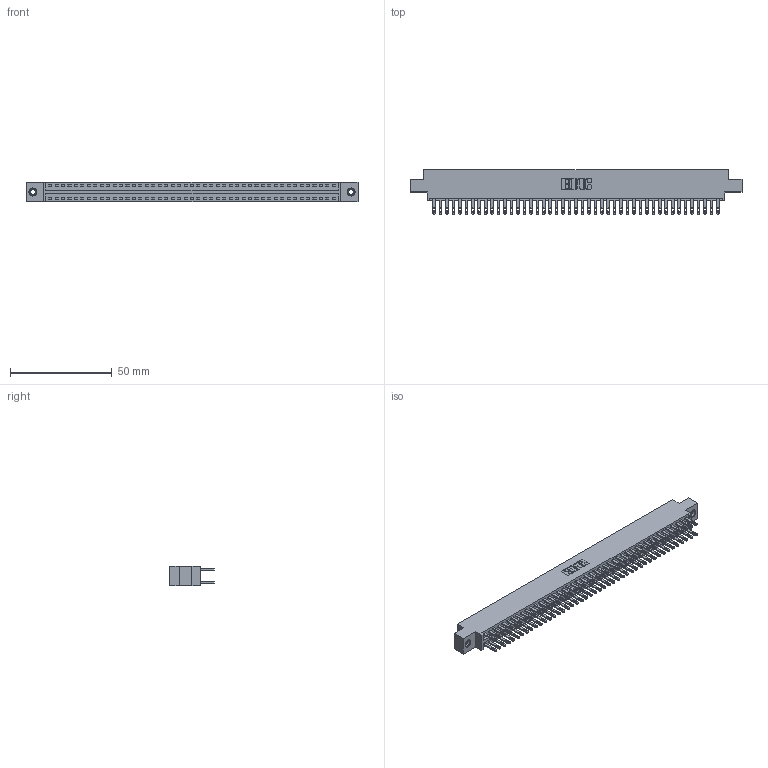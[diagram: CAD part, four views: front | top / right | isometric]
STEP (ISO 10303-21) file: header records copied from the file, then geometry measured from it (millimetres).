
FILE_DESCRIPTION (( 'STEP AP203' ), '1' );
FILE_NAME ('346-090-500-807.STEP', '2022-05-26T02:54:39', ( '' ), ( '' ), 'SwSTEP 2.0', 'SolidWorks 2020', '' );
FILE_SCHEMA (( 'CONFIG_CONTROL_DESIGN' ));
Length unit declared in the file: inch
Products named in the file (4): 346 Part_0.170 Offset - 0.156 Dia-TI; 345-292-001_345-293-100; 345-250-001_345-250-005-103; 346-090-500-807
Assembly tree (93 placements, depth 2):
  346-090-500-807
    346 Part_0.170 Offset - 0.156 Dia-TI
    345-292-001_345-293-100  x90
    345-250-001_345-250-005-103  x2
Bounding box: 163.45 x 21.84 x 9.4 mm (x, y, z)
Volume: 16068.5 mm3; surface area: 23289.8 mm2
Topology: 93 solids, 93 shells, 4506 faces, 13707 edges, 9130 vertices
Faces by surface type: plane 2722, cylinder 1768, cone 12, torus 4
Entity records: 30212 total; most frequent: CARTESIAN_POINT 4959, ORIENTED_EDGE 4886, DIRECTION 4449, EDGE_CURVE 2443, VECTOR 2107, LINE 2107, VERTEX_POINT 1624, AXIS2_PLACEMENT_3D 1171
